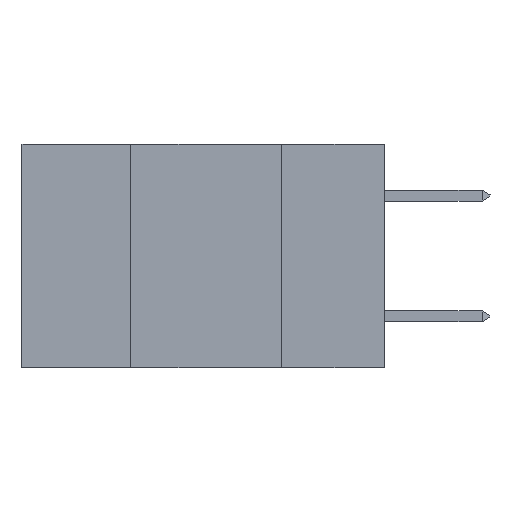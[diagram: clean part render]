
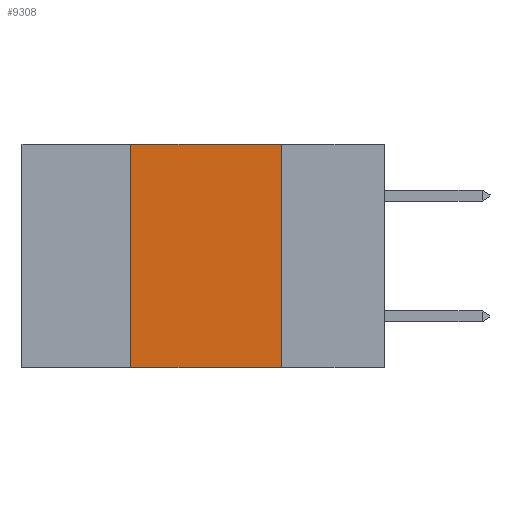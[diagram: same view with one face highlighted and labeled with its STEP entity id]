
A CAD part, left-side view. The second image highlights one B-rep face of the part: STEP entity #9308.
In plain terms, the highlighted planar face has unit normal (-1, 0, 0).
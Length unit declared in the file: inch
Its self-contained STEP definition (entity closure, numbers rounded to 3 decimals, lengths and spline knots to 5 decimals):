
#167 = VECTOR ( 'NONE', #12844, 39.37008 ) ;
#1273 = VERTEX_POINT ( 'NONE', #18993 ) ;
#3277 = EDGE_CURVE ( 'NONE', #6576, #24669, #21100, .T. ) ;
#3510 = PLANE ( 'NONE',  #13386 ) ;
#4787 = CARTESIAN_POINT ( 'NONE',  ( 0., 0.17, 0. ) ) ;
#4983 = CARTESIAN_POINT ( 'NONE',  ( 0., 0.42, 0. ) ) ;
#5718 = EDGE_CURVE ( 'NONE', #24669, #20202, #23088, .T. ) ;
#6217 = EDGE_CURVE ( 'NONE', #20202, #1273, #15709, .T. ) ;
#6576 = VERTEX_POINT ( 'NONE', #20184 ) ;
#7067 = DIRECTION ( 'NONE',  ( 0., -1., 0. ) ) ;
#9249 = LINE ( 'NONE', #19738, #25268 ) ;
#9308 = ADVANCED_FACE ( 'NONE', ( #24272 ), #3510, .F. ) ;
#10668 = DIRECTION ( 'NONE',  ( 0., 0., -1. ) ) ;
#11377 = VECTOR ( 'NONE', #10668, 39.37008 ) ;
#11446 = ORIENTED_EDGE ( 'NONE', *, *, #3277, .F. ) ;
#12021 = VECTOR ( 'NONE', #7067, 39.37008 ) ;
#12844 = DIRECTION ( 'NONE',  ( 0., 0., 1. ) ) ;
#13205 = ORIENTED_EDGE ( 'NONE', *, *, #5718, .F. ) ;
#13386 = AXIS2_PLACEMENT_3D ( 'NONE', #23162, #23792, #20637 ) ;
#13854 = EDGE_LOOP ( 'NONE', ( #16920, #13205, #11446, #17733 ) ) ;
#15452 = DIRECTION ( 'NONE',  ( 0., -1., 0. ) ) ;
#15709 = LINE ( 'NONE', #4787, #11377 ) ;
#16817 = CARTESIAN_POINT ( 'NONE',  ( 0., 0.42, 0. ) ) ;
#16920 = ORIENTED_EDGE ( 'NONE', *, *, #6217, .F. ) ;
#17733 = ORIENTED_EDGE ( 'NONE', *, *, #20939, .T. ) ;
#18993 = CARTESIAN_POINT ( 'NONE',  ( 0., 0.17, -0.37 ) ) ;
#19537 = CARTESIAN_POINT ( 'NONE',  ( 0., 0.17, 0. ) ) ;
#19738 = CARTESIAN_POINT ( 'NONE',  ( 0., 0.6, -0.37 ) ) ;
#20184 = CARTESIAN_POINT ( 'NONE',  ( 0., 0.42, -0.37 ) ) ;
#20202 = VERTEX_POINT ( 'NONE', #19537 ) ;
#20637 = DIRECTION ( 'NONE',  ( 0., 0., -1. ) ) ;
#20939 = EDGE_CURVE ( 'NONE', #6576, #1273, #9249, .T. ) ;
#21100 = LINE ( 'NONE', #4983, #167 ) ;
#22130 = CARTESIAN_POINT ( 'NONE',  ( 0., 0.6, 0. ) ) ;
#23088 = LINE ( 'NONE', #22130, #12021 ) ;
#23162 = CARTESIAN_POINT ( 'NONE',  ( 0., 0.6, 0. ) ) ;
#23792 = DIRECTION ( 'NONE',  ( 1., 0., 0. ) ) ;
#24272 = FACE_OUTER_BOUND ( 'NONE', #13854, .T. ) ;
#24669 = VERTEX_POINT ( 'NONE', #16817 ) ;
#25268 = VECTOR ( 'NONE', #15452, 39.37008 ) ;
